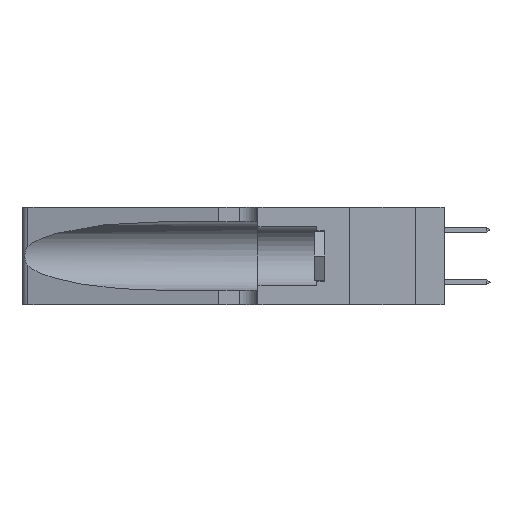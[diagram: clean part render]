
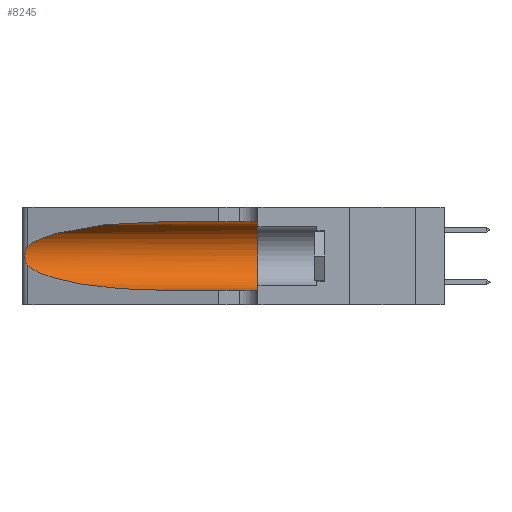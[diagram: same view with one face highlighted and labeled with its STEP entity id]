
A CAD part, left-side view. The second image highlights one B-rep face of the part: STEP entity #8245.
In plain terms, the highlighted cylindrical face has radius 3.308 mm (diameter 6.617 mm), a partial arc.
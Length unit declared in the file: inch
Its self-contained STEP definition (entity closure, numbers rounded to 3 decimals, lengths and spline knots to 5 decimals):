
#1163 = DIRECTION ( 'NONE',  ( 0., 0., -1. ) ) ;
#1266 = VERTEX_POINT ( 'NONE', #3553 ) ;
#1393 = AXIS2_PLACEMENT_3D ( 'NONE', #17962, #15275, #1163 ) ;
#1980 = CARTESIAN_POINT ( 'NONE',  ( 0.2373, 1.15595, 0.28018 ) ) ;
#2137 = DIRECTION ( 'NONE',  ( 0., 1., 0. ) ) ;
#2176 = ORIENTED_EDGE ( 'NONE', *, *, #12058, .F. ) ;
#2932 = ORIENTED_EDGE ( 'NONE', *, *, #15806, .T. ) ;
#3520 =( BOUNDED_CURVE ( )  B_SPLINE_CURVE ( 3, ( #11206, #7589, #1980, #21752 ),
 .UNSPECIFIED., .F., .F. ) 
 B_SPLINE_CURVE_WITH_KNOTS ( ( 4, 4 ),
 ( 1.5708, 2.84003 ),
 .UNSPECIFIED. ) 
 CURVE ( )  GEOMETRIC_REPRESENTATION_ITEM ( )  RATIONAL_B_SPLINE_CURVE ( ( 1., 0.87, 0.87, 1. ) ) 
 REPRESENTATION_ITEM ( '' )  );
#3553 = CARTESIAN_POINT ( 'NONE',  ( 0.25487, 1.22718, 0.22369 ) ) ;
#3931 = CARTESIAN_POINT ( 'NONE',  ( 0.25856, 1.23593, 0.16098 ) ) ;
#4397 = CARTESIAN_POINT ( 'NONE',  ( 0.25487, 1.22718, 0.14631 ) ) ;
#4433 = FACE_OUTER_BOUND ( 'NONE', #7743, .T. ) ;
#4816 = VERTEX_POINT ( 'NONE', #9990 ) ;
#6513 = CARTESIAN_POINT ( 'NONE',  ( 0.25487, 1.22718, 0.22369 ) ) ;
#6706 =( BOUNDED_CURVE ( )  B_SPLINE_CURVE ( 3, ( #4397, #12787, #15876, #10440 ),
 .UNSPECIFIED., .F., .F. ) 
 B_SPLINE_CURVE_WITH_KNOTS ( ( 4, 4 ),
 ( 3.44316, 4.71239 ),
 .UNSPECIFIED. ) 
 CURVE ( )  GEOMETRIC_REPRESENTATION_ITEM ( )  RATIONAL_B_SPLINE_CURVE ( ( 1., 0.87, 0.87, 1. ) ) 
 REPRESENTATION_ITEM ( '' )  );
#6771 = CARTESIAN_POINT ( 'NONE',  ( 0.25639, 1.23186, 0.15144 ) ) ;
#7483 = CARTESIAN_POINT ( 'NONE',  ( 0.25487, 1.22718, 0.14631 ) ) ;
#7589 = CARTESIAN_POINT ( 'NONE',  ( 0.18966, 0.96281, 0.31525 ) ) ;
#7743 = EDGE_LOOP ( 'NONE', ( #2932, #20167, #27628, #24952, #17462, #2176 ) ) ;
#8245 = ADVANCED_FACE ( 'NONE', ( #4433 ), #15956, .F. ) ;
#8488 = B_SPLINE_CURVE_WITH_KNOTS ( 'NONE', 3,
 ( #6513, #23315, #31992, #34946, #9218, #15029, #17845, #17967, #20813, #3931, #23667, #6771, #29372, #12435 ),
 .UNSPECIFIED., .F., .F.,
 ( 4, 2, 2, 2, 2, 2, 4 ),
 ( 0., 0.00027, 0.00053, 0.00107, 0.0016, 0.00187, 0.00214 ),
 .UNSPECIFIED. ) ;
#9218 = CARTESIAN_POINT ( 'NONE',  ( 0.25854, 1.2359, 0.20912 ) ) ;
#9990 = CARTESIAN_POINT ( 'NONE',  ( 0.1305, 0.35, 0.05475 ) ) ;
#10440 = CARTESIAN_POINT ( 'NONE',  ( 0.1305, 0.72297, 0.05475 ) ) ;
#11206 = CARTESIAN_POINT ( 'NONE',  ( 0.1305, 0.72297, 0.31525 ) ) ;
#12058 = EDGE_CURVE ( 'NONE', #13677, #14174, #28461, .T. ) ;
#12435 = CARTESIAN_POINT ( 'NONE',  ( 0.25487, 1.22718, 0.14631 ) ) ;
#12787 = CARTESIAN_POINT ( 'NONE',  ( 0.2373, 1.15595, 0.08982 ) ) ;
#13296 = EDGE_CURVE ( 'NONE', #29524, #14954, #6706, .T. ) ;
#13677 = VERTEX_POINT ( 'NONE', #19309 ) ;
#14174 = VERTEX_POINT ( 'NONE', #32103 ) ;
#14954 = VERTEX_POINT ( 'NONE', #32053 ) ;
#15029 = CARTESIAN_POINT ( 'NONE',  ( 0.26018, 1.23835, 0.19895 ) ) ;
#15275 = DIRECTION ( 'NONE',  ( 0., -1., 0. ) ) ;
#15806 = EDGE_CURVE ( 'NONE', #13677, #1266, #3520, .T. ) ;
#15876 = CARTESIAN_POINT ( 'NONE',  ( 0.18966, 0.96281, 0.05475 ) ) ;
#15956 = CYLINDRICAL_SURFACE ( 'NONE', #1393, 0.13025 ) ;
#17462 = ORIENTED_EDGE ( 'NONE', *, *, #23262, .F. ) ;
#17845 = CARTESIAN_POINT ( 'NONE',  ( 0.26075, 1.23896, 0.19203 ) ) ;
#17962 = CARTESIAN_POINT ( 'NONE',  ( 0.1305, 1.61858, 0.185 ) ) ;
#17967 = CARTESIAN_POINT ( 'NONE',  ( 0.26075, 1.23896, 0.178 ) ) ;
#19034 = CARTESIAN_POINT ( 'NONE',  ( 0.1305, 0.35, 0.185 ) ) ;
#19309 = CARTESIAN_POINT ( 'NONE',  ( 0.1305, 0.72297, 0.31525 ) ) ;
#20167 = ORIENTED_EDGE ( 'NONE', *, *, #32284, .T. ) ;
#20813 = CARTESIAN_POINT ( 'NONE',  ( 0.26017, 1.23833, 0.17102 ) ) ;
#21638 = LINE ( 'NONE', #33803, #27395 ) ;
#21752 = CARTESIAN_POINT ( 'NONE',  ( 0.25487, 1.22718, 0.22369 ) ) ;
#21866 = DIRECTION ( 'NONE',  ( 0., -1., 0. ) ) ;
#23262 = EDGE_CURVE ( 'NONE', #14174, #4816, #25852, .T. ) ;
#23315 = CARTESIAN_POINT ( 'NONE',  ( 0.25555, 1.22994, 0.2215 ) ) ;
#23667 = CARTESIAN_POINT ( 'NONE',  ( 0.25789, 1.23486, 0.15765 ) ) ;
#24952 = ORIENTED_EDGE ( 'NONE', *, *, #26903, .T. ) ;
#25852 = CIRCLE ( 'NONE', #35572, 0.13025 ) ;
#26903 = EDGE_CURVE ( 'NONE', #14954, #4816, #21638, .T. ) ;
#27055 = CARTESIAN_POINT ( 'NONE',  ( 0.1305, 1.61858, 0.31525 ) ) ;
#27395 = VECTOR ( 'NONE', #30043, 39.37008 ) ;
#27628 = ORIENTED_EDGE ( 'NONE', *, *, #13296, .T. ) ;
#28461 = LINE ( 'NONE', #27055, #35523 ) ;
#29372 = CARTESIAN_POINT ( 'NONE',  ( 0.25555, 1.22993, 0.14849 ) ) ;
#29524 = VERTEX_POINT ( 'NONE', #7483 ) ;
#30043 = DIRECTION ( 'NONE',  ( 0., -1., 0. ) ) ;
#31992 = CARTESIAN_POINT ( 'NONE',  ( 0.25639, 1.23184, 0.21858 ) ) ;
#32053 = CARTESIAN_POINT ( 'NONE',  ( 0.1305, 0.72297, 0.05475 ) ) ;
#32103 = CARTESIAN_POINT ( 'NONE',  ( 0.1305, 0.35, 0.31525 ) ) ;
#32284 = EDGE_CURVE ( 'NONE', #1266, #29524, #8488, .T. ) ;
#33803 = CARTESIAN_POINT ( 'NONE',  ( 0.1305, 1.61858, 0.05475 ) ) ;
#33809 = DIRECTION ( 'NONE',  ( 0., 0., 1. ) ) ;
#34946 = CARTESIAN_POINT ( 'NONE',  ( 0.25787, 1.23484, 0.2124 ) ) ;
#35523 = VECTOR ( 'NONE', #21866, 39.37008 ) ;
#35572 = AXIS2_PLACEMENT_3D ( 'NONE', #19034, #2137, #33809 ) ;
